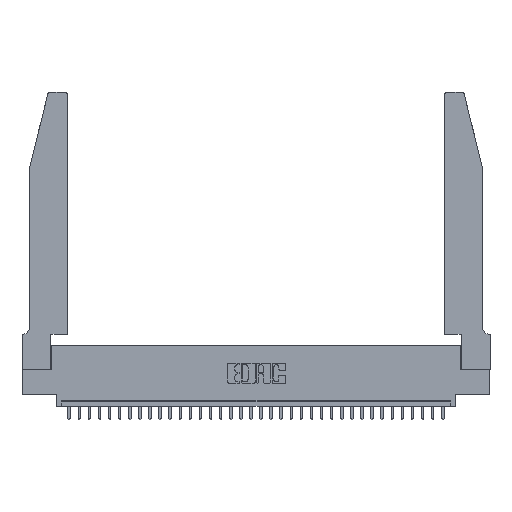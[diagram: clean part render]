
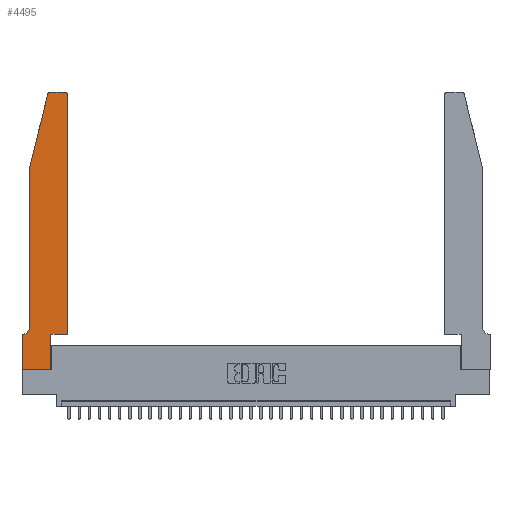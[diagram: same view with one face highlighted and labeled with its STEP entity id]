
A CAD part, top view. The second image highlights one B-rep face of the part: STEP entity #4495.
In plain terms, the highlighted planar face has unit normal (0, 0, 1).
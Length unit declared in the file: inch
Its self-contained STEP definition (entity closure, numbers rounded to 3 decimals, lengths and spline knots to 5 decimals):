
#320 = EDGE_CURVE ( 'NONE', #2680, #14566, #27712, .T. ) ;
#450 = DIRECTION ( 'NONE',  ( -1., 0., 0. ) ) ;
#578 = CARTESIAN_POINT ( 'NONE',  ( 0.4505, 2.72, 0.37 ) ) ;
#599 = VERTEX_POINT ( 'NONE', #8498 ) ;
#1028 = CARTESIAN_POINT ( 'NONE',  ( 0.0755, 2., 0.37 ) ) ;
#1414 = CARTESIAN_POINT ( 'NONE',  ( 0., 0.35, 0.37 ) ) ;
#1723 = DIRECTION ( 'NONE',  ( 1., 0., 0. ) ) ;
#2097 = VERTEX_POINT ( 'NONE', #578 ) ;
#2498 = DIRECTION ( 'NONE',  ( 1., 0., 0. ) ) ;
#2615 = CARTESIAN_POINT ( 'NONE',  ( 0.0055, 0.35, 0.37 ) ) ;
#2680 = VERTEX_POINT ( 'NONE', #32119 ) ;
#3094 = CARTESIAN_POINT ( 'NONE',  ( 0.4505, 0.35, 0.37 ) ) ;
#3784 = DIRECTION ( 'NONE',  ( -0.239, -0.971, 0. ) ) ;
#3959 = DIRECTION ( 'NONE',  ( 1., 0., 0. ) ) ;
#4002 = CARTESIAN_POINT ( 'NONE',  ( 0.0755, 0.42, 0.37 ) ) ;
#4119 = CARTESIAN_POINT ( 'NONE',  ( 0.2865, 0.35, 0.37 ) ) ;
#4344 = DIRECTION ( 'NONE',  ( 0., 1., 0. ) ) ;
#4495 = ADVANCED_FACE ( 'NONE', ( #18402 ), #18540, .T. ) ;
#4953 = AXIS2_PLACEMENT_3D ( 'NONE', #18204, #23749, #2498 ) ;
#5842 = DIRECTION ( 'NONE',  ( 1., 0., 0. ) ) ;
#6533 = ORIENTED_EDGE ( 'NONE', *, *, #18544, .T. ) ;
#6820 = CARTESIAN_POINT ( 'NONE',  ( 0.4205, 2.75, 0.37 ) ) ;
#6886 = DIRECTION ( 'NONE',  ( -1., 0., 0. ) ) ;
#7097 = ORIENTED_EDGE ( 'NONE', *, *, #19619, .T. ) ;
#7176 = AXIS2_PLACEMENT_3D ( 'NONE', #8166, #16071, #450 ) ;
#7681 = VERTEX_POINT ( 'NONE', #1028 ) ;
#7842 = EDGE_CURVE ( 'NONE', #20206, #30000, #29357, .T. ) ;
#7867 = DIRECTION ( 'NONE',  ( 0., -1., 0. ) ) ;
#8166 = CARTESIAN_POINT ( 'NONE',  ( 0.0055, 0.42, 0.37 ) ) ;
#8498 = CARTESIAN_POINT ( 'NONE',  ( 0., 0., 0.37 ) ) ;
#9241 = VECTOR ( 'NONE', #3959, 39.37008 ) ;
#9368 = CARTESIAN_POINT ( 'NONE',  ( 0., 0., 0.37 ) ) ;
#9377 = ORIENTED_EDGE ( 'NONE', *, *, #320, .T. ) ;
#9424 = ORIENTED_EDGE ( 'NONE', *, *, #34048, .T. ) ;
#9512 = LINE ( 'NONE', #14800, #16035 ) ;
#9648 = LINE ( 'NONE', #13021, #26110 ) ;
#9723 = AXIS2_PLACEMENT_3D ( 'NONE', #22531, #28529, #5842 ) ;
#10659 = EDGE_CURVE ( 'NONE', #7681, #30608, #9648, .T. ) ;
#11587 = LINE ( 'NONE', #27577, #26813 ) ;
#11652 = VERTEX_POINT ( 'NONE', #6820 ) ;
#11659 = CARTESIAN_POINT ( 'NONE',  ( 0.25487, 2.72718, 0.37 ) ) ;
#12107 = CIRCLE ( 'NONE', #7176, 0.07 ) ;
#12367 = ORIENTED_EDGE ( 'NONE', *, *, #29553, .T. ) ;
#12372 = CARTESIAN_POINT ( 'NONE',  ( 0.4205, 2.72, 0.37 ) ) ;
#13021 = CARTESIAN_POINT ( 'NONE',  ( 0.0755, 2., 0.37 ) ) ;
#13298 = VERTEX_POINT ( 'NONE', #1414 ) ;
#13457 = VERTEX_POINT ( 'NONE', #18741 ) ;
#14364 = CARTESIAN_POINT ( 'NONE',  ( 0.0755, 0.35, 0.37 ) ) ;
#14566 = VERTEX_POINT ( 'NONE', #11659 ) ;
#14800 = CARTESIAN_POINT ( 'NONE',  ( 0.2605, 2.75, 0.37 ) ) ;
#15131 = VECTOR ( 'NONE', #26760, 39.37008 ) ;
#15955 = LINE ( 'NONE', #3094, #15131 ) ;
#16035 = VECTOR ( 'NONE', #28305, 39.37008 ) ;
#16062 = AXIS2_PLACEMENT_3D ( 'NONE', #12372, #27931, #1723 ) ;
#16071 = DIRECTION ( 'NONE',  ( 0., 0., -1. ) ) ;
#16186 = LINE ( 'NONE', #9368, #9241 ) ;
#16490 = EDGE_CURVE ( 'NONE', #30608, #30843, #12107, .T. ) ;
#16686 = CARTESIAN_POINT ( 'NONE',  ( 0.4505, 0.35, 0.37 ) ) ;
#16967 = EDGE_CURVE ( 'NONE', #30843, #13298, #21552, .T. ) ;
#17431 = LINE ( 'NONE', #16686, #23246 ) ;
#18204 = CARTESIAN_POINT ( 'NONE',  ( 0., 0.35, 0.37 ) ) ;
#18402 = FACE_OUTER_BOUND ( 'NONE', #20881, .T. ) ;
#18528 = ORIENTED_EDGE ( 'NONE', *, *, #10659, .T. ) ;
#18540 = PLANE ( 'NONE',  #4953 ) ;
#18544 = EDGE_CURVE ( 'NONE', #11652, #2680, #9512, .T. ) ;
#18741 = CARTESIAN_POINT ( 'NONE',  ( 0.4505, 0.35, 0.37 ) ) ;
#18856 = ORIENTED_EDGE ( 'NONE', *, *, #21761, .T. ) ;
#19434 = CIRCLE ( 'NONE', #16062, 0.03 ) ;
#19619 = EDGE_CURVE ( 'NONE', #30000, #13457, #17431, .T. ) ;
#20033 = ORIENTED_EDGE ( 'NONE', *, *, #16967, .T. ) ;
#20206 = VERTEX_POINT ( 'NONE', #31282 ) ;
#20452 = VECTOR ( 'NONE', #3784, 39.37008 ) ;
#20881 = EDGE_LOOP ( 'NONE', ( #6533, #9377, #12367, #18528, #24238, #20033, #18856, #33337, #28981, #7097, #9424, #21517 ) ) ;
#21517 = ORIENTED_EDGE ( 'NONE', *, *, #31993, .T. ) ;
#21552 = LINE ( 'NONE', #14364, #26897 ) ;
#21761 = EDGE_CURVE ( 'NONE', #13298, #599, #11587, .T. ) ;
#22531 = CARTESIAN_POINT ( 'NONE',  ( 0.284, 2.72, 0.37 ) ) ;
#22754 = VECTOR ( 'NONE', #4344, 39.37008 ) ;
#23246 = VECTOR ( 'NONE', #32651, 39.37008 ) ;
#23749 = DIRECTION ( 'NONE',  ( 0., 0., 1. ) ) ;
#24238 = ORIENTED_EDGE ( 'NONE', *, *, #16490, .T. ) ;
#26110 = VECTOR ( 'NONE', #7867, 39.37008 ) ;
#26760 = DIRECTION ( 'NONE',  ( 0., 1., 0. ) ) ;
#26813 = VECTOR ( 'NONE', #30340, 39.37008 ) ;
#26897 = VECTOR ( 'NONE', #6886, 39.37008 ) ;
#27431 = LINE ( 'NONE', #32478, #20452 ) ;
#27577 = CARTESIAN_POINT ( 'NONE',  ( 0., 0., 0.37 ) ) ;
#27712 = CIRCLE ( 'NONE', #9723, 0.03 ) ;
#27931 = DIRECTION ( 'NONE',  ( 0., 0., 1. ) ) ;
#28305 = DIRECTION ( 'NONE',  ( -1., 0., 0. ) ) ;
#28529 = DIRECTION ( 'NONE',  ( 0., 0., 1. ) ) ;
#28944 = CARTESIAN_POINT ( 'NONE',  ( 0.2865, 0.35, 0.37 ) ) ;
#28981 = ORIENTED_EDGE ( 'NONE', *, *, #7842, .T. ) ;
#29357 = LINE ( 'NONE', #4119, #22754 ) ;
#29553 = EDGE_CURVE ( 'NONE', #14566, #7681, #27431, .T. ) ;
#30000 = VERTEX_POINT ( 'NONE', #28944 ) ;
#30340 = DIRECTION ( 'NONE',  ( 0., -1., 0. ) ) ;
#30608 = VERTEX_POINT ( 'NONE', #4002 ) ;
#30843 = VERTEX_POINT ( 'NONE', #2615 ) ;
#31120 = EDGE_CURVE ( 'NONE', #599, #20206, #16186, .T. ) ;
#31282 = CARTESIAN_POINT ( 'NONE',  ( 0.2865, 0., 0.37 ) ) ;
#31993 = EDGE_CURVE ( 'NONE', #2097, #11652, #19434, .T. ) ;
#32119 = CARTESIAN_POINT ( 'NONE',  ( 0.284, 2.75, 0.37 ) ) ;
#32478 = CARTESIAN_POINT ( 'NONE',  ( 0.0755, 2., 0.37 ) ) ;
#32651 = DIRECTION ( 'NONE',  ( 1., 0., 0. ) ) ;
#33337 = ORIENTED_EDGE ( 'NONE', *, *, #31120, .T. ) ;
#34048 = EDGE_CURVE ( 'NONE', #13457, #2097, #15955, .T. ) ;
